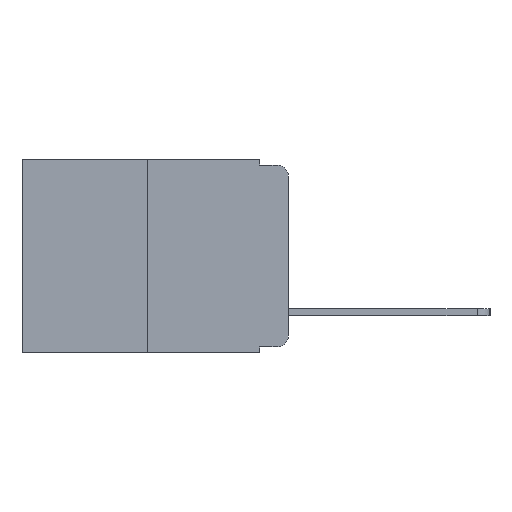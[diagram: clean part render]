
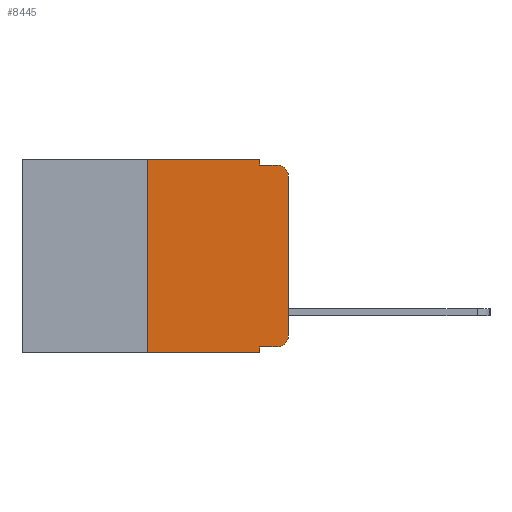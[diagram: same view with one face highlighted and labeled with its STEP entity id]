
A CAD part, left-side view. The second image highlights one B-rep face of the part: STEP entity #8445.
In plain terms, the highlighted planar face has unit normal (-1, 0, 0).
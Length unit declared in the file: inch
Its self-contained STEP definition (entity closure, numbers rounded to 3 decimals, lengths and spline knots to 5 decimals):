
#177 = ORIENTED_EDGE ( 'NONE', *, *, #910, .F. ) ;
#255 = EDGE_CURVE ( 'NONE', #6837, #9280, #6495, .T. ) ;
#398 = CARTESIAN_POINT ( 'NONE',  ( 0., 0.25, 0. ) ) ;
#407 = CARTESIAN_POINT ( 'NONE',  ( 0., 0.02, -0.333 ) ) ;
#491 = ORIENTED_EDGE ( 'NONE', *, *, #10425, .T. ) ;
#910 = EDGE_CURVE ( 'NONE', #1290, #8356, #10441, .T. ) ;
#1069 = VERTEX_POINT ( 'NONE', #3476 ) ;
#1154 = EDGE_CURVE ( 'NONE', #1069, #10958, #10564, .T. ) ;
#1216 = DIRECTION ( 'NONE',  ( 1., 0., 0. ) ) ;
#1248 = ORIENTED_EDGE ( 'NONE', *, *, #7030, .F. ) ;
#1290 = VERTEX_POINT ( 'NONE', #1571 ) ;
#1309 = DIRECTION ( 'NONE',  ( 0., 0., -1. ) ) ;
#1571 = CARTESIAN_POINT ( 'NONE',  ( 0., 0.051, -0.333 ) ) ;
#1958 = LINE ( 'NONE', #6017, #6423 ) ;
#2127 = AXIS2_PLACEMENT_3D ( 'NONE', #6620, #1216, #7474 ) ;
#2189 = EDGE_CURVE ( 'NONE', #10333, #9671, #8550, .T. ) ;
#2293 = VECTOR ( 'NONE', #5112, 39.37008 ) ;
#2741 = VECTOR ( 'NONE', #8957, 39.37008 ) ;
#2825 = CARTESIAN_POINT ( 'NONE',  ( 0., 0.051, 0. ) ) ;
#3050 = VERTEX_POINT ( 'NONE', #2825 ) ;
#3452 = EDGE_CURVE ( 'NONE', #9280, #10333, #3455, .T. ) ;
#3455 = LINE ( 'NONE', #6720, #9859 ) ;
#3476 = CARTESIAN_POINT ( 'NONE',  ( 0., 0.25, -0.343 ) ) ;
#3594 = EDGE_CURVE ( 'NONE', #10958, #3050, #1958, .T. ) ;
#4004 = CARTESIAN_POINT ( 'NONE',  ( 0., 0.25, 0. ) ) ;
#4078 = FACE_OUTER_BOUND ( 'NONE', #4296, .T. ) ;
#4296 = EDGE_LOOP ( 'NONE', ( #7542, #8311, #1248, #10697, #9042, #10975, #7164, #177, #491, #9763 ) ) ;
#4321 = AXIS2_PLACEMENT_3D ( 'NONE', #9762, #9770, #9785 ) ;
#4608 = CARTESIAN_POINT ( 'NONE',  ( 0., 0.051, -0.01 ) ) ;
#4830 = LINE ( 'NONE', #11120, #8737 ) ;
#4923 = PLANE ( 'NONE',  #2127 ) ;
#5044 = DIRECTION ( 'NONE',  ( 0., -1., 0. ) ) ;
#5112 = DIRECTION ( 'NONE',  ( 0., -1., 0. ) ) ;
#5132 = CARTESIAN_POINT ( 'NONE',  ( 0., 0.02, -0.313 ) ) ;
#5398 = LINE ( 'NONE', #5630, #2741 ) ;
#5630 = CARTESIAN_POINT ( 'NONE',  ( 0., 0.473, -0.343 ) ) ;
#5700 = VECTOR ( 'NONE', #1309, 39.37008 ) ;
#6017 = CARTESIAN_POINT ( 'NONE',  ( 0., 0.473, 0. ) ) ;
#6081 = VECTOR ( 'NONE', #8238, 39.37008 ) ;
#6165 = DIRECTION ( 'NONE',  ( 0., -1., 0. ) ) ;
#6423 = VECTOR ( 'NONE', #5044, 39.37008 ) ;
#6480 = DIRECTION ( 'NONE',  ( 0., 0., 1. ) ) ;
#6495 = CIRCLE ( 'NONE', #10201, 0.02 ) ;
#6620 = CARTESIAN_POINT ( 'NONE',  ( 0., 0.473, 0. ) ) ;
#6706 = CARTESIAN_POINT ( 'NONE',  ( 0., 0.051, 0. ) ) ;
#6720 = CARTESIAN_POINT ( 'NONE',  ( 0., 0., 0. ) ) ;
#6762 = DIRECTION ( 'NONE',  ( 0., 0., 1. ) ) ;
#6837 = VERTEX_POINT ( 'NONE', #407 ) ;
#6928 = CARTESIAN_POINT ( 'NONE',  ( 0., 0., -0.313 ) ) ;
#7030 = EDGE_CURVE ( 'NONE', #8890, #9671, #4830, .T. ) ;
#7164 = ORIENTED_EDGE ( 'NONE', *, *, #10187, .T. ) ;
#7312 = DIRECTION ( 'NONE',  ( 0., 0., -1. ) ) ;
#7474 = DIRECTION ( 'NONE',  ( 0., 0., -1. ) ) ;
#7542 = ORIENTED_EDGE ( 'NONE', *, *, #3452, .T. ) ;
#7671 = CARTESIAN_POINT ( 'NONE',  ( 0., 0.051, -0.333 ) ) ;
#7807 = CARTESIAN_POINT ( 'NONE',  ( 0., 0.051, 0. ) ) ;
#8181 = VECTOR ( 'NONE', #6480, 39.37008 ) ;
#8238 = DIRECTION ( 'NONE',  ( 0., 0., -1. ) ) ;
#8311 = ORIENTED_EDGE ( 'NONE', *, *, #2189, .T. ) ;
#8356 = VERTEX_POINT ( 'NONE', #10537 ) ;
#8384 = CARTESIAN_POINT ( 'NONE',  ( 0., 0., -0.03 ) ) ;
#8445 = ADVANCED_FACE ( 'NONE', ( #4078 ), #4923, .F. ) ;
#8550 = CIRCLE ( 'NONE', #4321, 0.02 ) ;
#8665 = EDGE_CURVE ( 'NONE', #3050, #8890, #9530, .T. ) ;
#8737 = VECTOR ( 'NONE', #6165, 39.37008 ) ;
#8890 = VERTEX_POINT ( 'NONE', #4608 ) ;
#8893 = LINE ( 'NONE', #7671, #2293 ) ;
#8957 = DIRECTION ( 'NONE',  ( 0., -1., 0. ) ) ;
#9042 = ORIENTED_EDGE ( 'NONE', *, *, #3594, .F. ) ;
#9280 = VERTEX_POINT ( 'NONE', #6928 ) ;
#9530 = LINE ( 'NONE', #6706, #5700 ) ;
#9671 = VERTEX_POINT ( 'NONE', #10671 ) ;
#9762 = CARTESIAN_POINT ( 'NONE',  ( 0., 0.02, -0.03 ) ) ;
#9763 = ORIENTED_EDGE ( 'NONE', *, *, #255, .T. ) ;
#9770 = DIRECTION ( 'NONE',  ( -1., 0., 0. ) ) ;
#9785 = DIRECTION ( 'NONE',  ( 0., 0., -1. ) ) ;
#9859 = VECTOR ( 'NONE', #6762, 39.37008 ) ;
#10187 = EDGE_CURVE ( 'NONE', #1069, #8356, #5398, .T. ) ;
#10201 = AXIS2_PLACEMENT_3D ( 'NONE', #5132, #11085, #7312 ) ;
#10333 = VERTEX_POINT ( 'NONE', #8384 ) ;
#10425 = EDGE_CURVE ( 'NONE', #1290, #6837, #8893, .T. ) ;
#10441 = LINE ( 'NONE', #7807, #6081 ) ;
#10537 = CARTESIAN_POINT ( 'NONE',  ( 0., 0.051, -0.343 ) ) ;
#10564 = LINE ( 'NONE', #4004, #8181 ) ;
#10671 = CARTESIAN_POINT ( 'NONE',  ( 0., 0.02, -0.01 ) ) ;
#10697 = ORIENTED_EDGE ( 'NONE', *, *, #8665, .F. ) ;
#10958 = VERTEX_POINT ( 'NONE', #398 ) ;
#10975 = ORIENTED_EDGE ( 'NONE', *, *, #1154, .F. ) ;
#11085 = DIRECTION ( 'NONE',  ( -1., 0., 0. ) ) ;
#11120 = CARTESIAN_POINT ( 'NONE',  ( 0., 0.051, -0.01 ) ) ;
